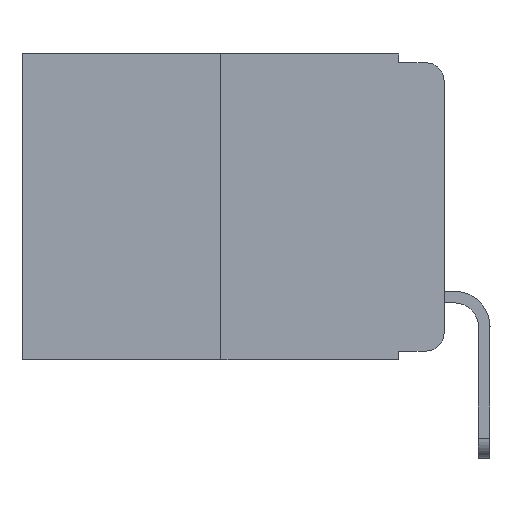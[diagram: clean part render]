
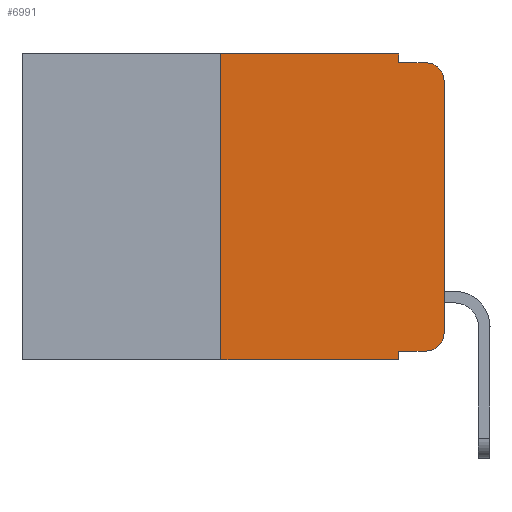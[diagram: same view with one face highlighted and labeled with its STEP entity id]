
A CAD part, left-side view. The second image highlights one B-rep face of the part: STEP entity #6991.
In plain terms, the highlighted planar face has unit normal (-1, 0, 0).
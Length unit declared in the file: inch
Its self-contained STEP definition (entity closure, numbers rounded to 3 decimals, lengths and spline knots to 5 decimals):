
#31 = ORIENTED_EDGE ( 'NONE', *, *, #20135, .T. ) ;
#37 = CARTESIAN_POINT ( 'NONE',  ( 0., 0., -0.313 ) ) ;
#359 = EDGE_CURVE ( 'NONE', #2521, #8019, #13660, .T. ) ;
#1249 = EDGE_CURVE ( 'NONE', #19010, #10250, #20470, .T. ) ;
#1699 = CARTESIAN_POINT ( 'NONE',  ( 0., 0.25, -0.343 ) ) ;
#1758 = VECTOR ( 'NONE', #9016, 39.37008 ) ;
#2118 = DIRECTION ( 'NONE',  ( 0., -1., 0. ) ) ;
#2521 = VERTEX_POINT ( 'NONE', #37 ) ;
#3119 = ORIENTED_EDGE ( 'NONE', *, *, #24792, .F. ) ;
#3411 = VERTEX_POINT ( 'NONE', #1699 ) ;
#3547 = AXIS2_PLACEMENT_3D ( 'NONE', #4591, #22814, #19073 ) ;
#3554 = CARTESIAN_POINT ( 'NONE',  ( 0., 0., 0. ) ) ;
#3729 = FACE_OUTER_BOUND ( 'NONE', #19348, .T. ) ;
#4023 = VERTEX_POINT ( 'NONE', #24921 ) ;
#4388 = CARTESIAN_POINT ( 'NONE',  ( 0., 0.473, -0.343 ) ) ;
#4485 = DIRECTION ( 'NONE',  ( 0., 0., 1. ) ) ;
#4591 = CARTESIAN_POINT ( 'NONE',  ( 0., 0.02, -0.03 ) ) ;
#4784 = LINE ( 'NONE', #4388, #15761 ) ;
#4974 = CARTESIAN_POINT ( 'NONE',  ( 0., 0.051, -0.01 ) ) ;
#5047 = DIRECTION ( 'NONE',  ( 0., 0., 1. ) ) ;
#5302 = DIRECTION ( 'NONE',  ( -1., 0., 0. ) ) ;
#5563 = LINE ( 'NONE', #10068, #7414 ) ;
#6766 = LINE ( 'NONE', #12606, #1758 ) ;
#6991 = ADVANCED_FACE ( 'NONE', ( #3729 ), #11824, .F. ) ;
#7166 = CARTESIAN_POINT ( 'NONE',  ( 0., 0.25, 0. ) ) ;
#7414 = VECTOR ( 'NONE', #19794, 39.37008 ) ;
#8019 = VERTEX_POINT ( 'NONE', #14133 ) ;
#8215 = VERTEX_POINT ( 'NONE', #23951 ) ;
#9016 = DIRECTION ( 'NONE',  ( 0., -1., 0. ) ) ;
#9182 = CARTESIAN_POINT ( 'NONE',  ( 0., 0.473, 0. ) ) ;
#9369 = CARTESIAN_POINT ( 'NONE',  ( 0., 0.051, -0.333 ) ) ;
#9903 = CARTESIAN_POINT ( 'NONE',  ( 0., 0.051, 0. ) ) ;
#10068 = CARTESIAN_POINT ( 'NONE',  ( 0., 0.051, 0. ) ) ;
#10250 = VERTEX_POINT ( 'NONE', #21761 ) ;
#10350 = LINE ( 'NONE', #15362, #13698 ) ;
#10978 = AXIS2_PLACEMENT_3D ( 'NONE', #25245, #5302, #17005 ) ;
#11824 = PLANE ( 'NONE',  #17193 ) ;
#12286 = CARTESIAN_POINT ( 'NONE',  ( 0., 0.02, -0.01 ) ) ;
#12501 = VECTOR ( 'NONE', #2118, 39.37008 ) ;
#12606 = CARTESIAN_POINT ( 'NONE',  ( 0., 0.473, 0. ) ) ;
#13065 = DIRECTION ( 'NONE',  ( 0., -1., 0. ) ) ;
#13660 = LINE ( 'NONE', #3554, #19582 ) ;
#13698 = VECTOR ( 'NONE', #17363, 39.37008 ) ;
#13758 = EDGE_CURVE ( 'NONE', #15250, #19103, #17453, .T. ) ;
#14133 = CARTESIAN_POINT ( 'NONE',  ( 0., 0., -0.03 ) ) ;
#15029 = EDGE_CURVE ( 'NONE', #10250, #2521, #24654, .T. ) ;
#15250 = VERTEX_POINT ( 'NONE', #15661 ) ;
#15292 = DIRECTION ( 'NONE',  ( 1., 0., 0. ) ) ;
#15362 = CARTESIAN_POINT ( 'NONE',  ( 0., 0.051, 0. ) ) ;
#15661 = CARTESIAN_POINT ( 'NONE',  ( 0., 0.051, -0.01 ) ) ;
#15761 = VECTOR ( 'NONE', #22998, 39.37008 ) ;
#16225 = CARTESIAN_POINT ( 'NONE',  ( 0., 0.051, -0.333 ) ) ;
#16898 = EDGE_CURVE ( 'NONE', #3411, #4023, #18162, .T. ) ;
#17005 = DIRECTION ( 'NONE',  ( 0., 0., -1. ) ) ;
#17193 = AXIS2_PLACEMENT_3D ( 'NONE', #9182, #15292, #23426 ) ;
#17363 = DIRECTION ( 'NONE',  ( 0., 0., -1. ) ) ;
#17411 = ORIENTED_EDGE ( 'NONE', *, *, #359, .T. ) ;
#17453 = LINE ( 'NONE', #4974, #22900 ) ;
#18162 = LINE ( 'NONE', #7166, #20823 ) ;
#18750 = ORIENTED_EDGE ( 'NONE', *, *, #15029, .T. ) ;
#18811 = EDGE_CURVE ( 'NONE', #22237, #15250, #10350, .T. ) ;
#18951 = ORIENTED_EDGE ( 'NONE', *, *, #20231, .F. ) ;
#19010 = VERTEX_POINT ( 'NONE', #9369 ) ;
#19073 = DIRECTION ( 'NONE',  ( 0., 0., -1. ) ) ;
#19103 = VERTEX_POINT ( 'NONE', #12286 ) ;
#19258 = CIRCLE ( 'NONE', #3547, 0.02 ) ;
#19348 = EDGE_LOOP ( 'NONE', ( #17411, #23338, #22033, #25169, #18951, #25586, #31, #3119, #19468, #18750 ) ) ;
#19468 = ORIENTED_EDGE ( 'NONE', *, *, #1249, .T. ) ;
#19582 = VECTOR ( 'NONE', #4485, 39.37008 ) ;
#19794 = DIRECTION ( 'NONE',  ( 0., 0., -1. ) ) ;
#20135 = EDGE_CURVE ( 'NONE', #3411, #8215, #4784, .T. ) ;
#20231 = EDGE_CURVE ( 'NONE', #4023, #22237, #6766, .T. ) ;
#20470 = LINE ( 'NONE', #16225, #12501 ) ;
#20823 = VECTOR ( 'NONE', #5047, 39.37008 ) ;
#21761 = CARTESIAN_POINT ( 'NONE',  ( 0., 0.02, -0.333 ) ) ;
#22033 = ORIENTED_EDGE ( 'NONE', *, *, #13758, .F. ) ;
#22237 = VERTEX_POINT ( 'NONE', #9903 ) ;
#22308 = EDGE_CURVE ( 'NONE', #8019, #19103, #19258, .T. ) ;
#22814 = DIRECTION ( 'NONE',  ( -1., 0., 0. ) ) ;
#22900 = VECTOR ( 'NONE', #13065, 39.37008 ) ;
#22998 = DIRECTION ( 'NONE',  ( 0., -1., 0. ) ) ;
#23338 = ORIENTED_EDGE ( 'NONE', *, *, #22308, .T. ) ;
#23426 = DIRECTION ( 'NONE',  ( 0., 0., -1. ) ) ;
#23951 = CARTESIAN_POINT ( 'NONE',  ( 0., 0.051, -0.343 ) ) ;
#24654 = CIRCLE ( 'NONE', #10978, 0.02 ) ;
#24792 = EDGE_CURVE ( 'NONE', #19010, #8215, #5563, .T. ) ;
#24921 = CARTESIAN_POINT ( 'NONE',  ( 0., 0.25, 0. ) ) ;
#25169 = ORIENTED_EDGE ( 'NONE', *, *, #18811, .F. ) ;
#25245 = CARTESIAN_POINT ( 'NONE',  ( 0., 0.02, -0.313 ) ) ;
#25586 = ORIENTED_EDGE ( 'NONE', *, *, #16898, .F. ) ;
